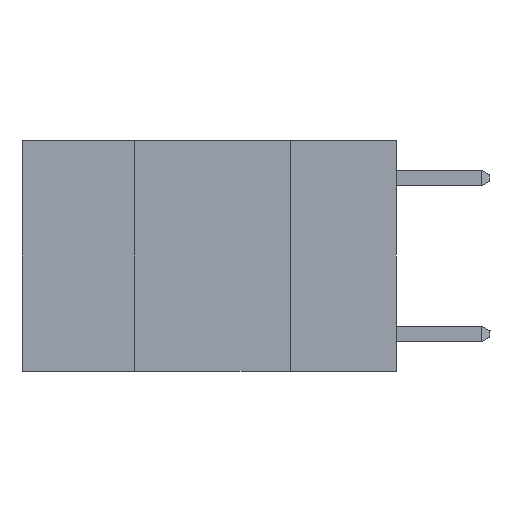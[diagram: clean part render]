
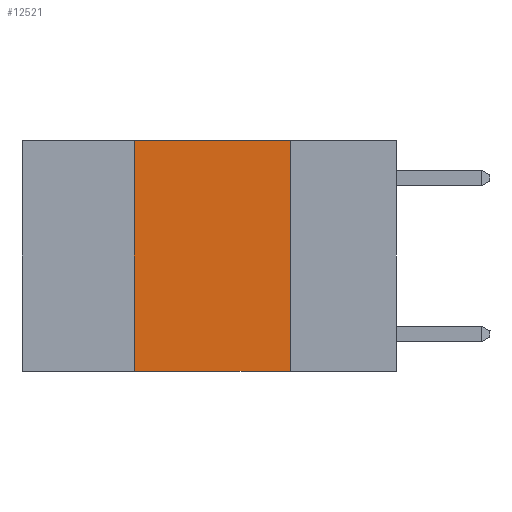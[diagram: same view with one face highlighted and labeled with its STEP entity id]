
A CAD part, left-side view. The second image highlights one B-rep face of the part: STEP entity #12521.
In plain terms, the highlighted planar face has unit normal (-1, 0, 0).
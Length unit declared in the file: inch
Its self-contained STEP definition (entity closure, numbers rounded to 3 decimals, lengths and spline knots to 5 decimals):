
#1039 = DIRECTION ( 'NONE',  ( 0., -1., 0. ) ) ;
#2225 = VECTOR ( 'NONE', #25345, 39.37008 ) ;
#4602 = DIRECTION ( 'NONE',  ( 0., -1., 0. ) ) ;
#4793 = EDGE_CURVE ( 'NONE', #11114, #27344, #6600, .T. ) ;
#6600 = LINE ( 'NONE', #28988, #23838 ) ;
#6808 = FACE_OUTER_BOUND ( 'NONE', #7672, .T. ) ;
#7672 = EDGE_LOOP ( 'NONE', ( #29712, #24950, #14705, #21653 ) ) ;
#9462 = PLANE ( 'NONE',  #22714 ) ;
#11114 = VERTEX_POINT ( 'NONE', #17862 ) ;
#11649 = CARTESIAN_POINT ( 'NONE',  ( 0., 0.17, -0.37 ) ) ;
#11840 = DIRECTION ( 'NONE',  ( 0., 0., -1. ) ) ;
#12386 = CARTESIAN_POINT ( 'NONE',  ( 0., 0.42, 0. ) ) ;
#12521 = ADVANCED_FACE ( 'NONE', ( #6808 ), #9462, .F. ) ;
#13565 = VECTOR ( 'NONE', #4602, 39.37008 ) ;
#13646 = VERTEX_POINT ( 'NONE', #23130 ) ;
#14705 = ORIENTED_EDGE ( 'NONE', *, *, #15365, .F. ) ;
#15365 = EDGE_CURVE ( 'NONE', #11114, #28292, #27159, .T. ) ;
#16125 = EDGE_CURVE ( 'NONE', #28292, #13646, #21261, .T. ) ;
#16358 = VECTOR ( 'NONE', #23430, 39.37008 ) ;
#17862 = CARTESIAN_POINT ( 'NONE',  ( 0., 0.42, -0.37 ) ) ;
#19428 = EDGE_CURVE ( 'NONE', #13646, #27344, #22568, .T. ) ;
#21086 = CARTESIAN_POINT ( 'NONE',  ( 0., 0.17, 0. ) ) ;
#21261 = LINE ( 'NONE', #30309, #13565 ) ;
#21653 = ORIENTED_EDGE ( 'NONE', *, *, #4793, .T. ) ;
#22568 = LINE ( 'NONE', #21086, #16358 ) ;
#22714 = AXIS2_PLACEMENT_3D ( 'NONE', #23493, #25834, #11840 ) ;
#23130 = CARTESIAN_POINT ( 'NONE',  ( 0., 0.17, 0. ) ) ;
#23430 = DIRECTION ( 'NONE',  ( 0., 0., -1. ) ) ;
#23493 = CARTESIAN_POINT ( 'NONE',  ( 0., 0.6, 0. ) ) ;
#23838 = VECTOR ( 'NONE', #1039, 39.37008 ) ;
#24950 = ORIENTED_EDGE ( 'NONE', *, *, #16125, .F. ) ;
#25345 = DIRECTION ( 'NONE',  ( 0., 0., 1. ) ) ;
#25834 = DIRECTION ( 'NONE',  ( 1., 0., 0. ) ) ;
#27159 = LINE ( 'NONE', #27709, #2225 ) ;
#27344 = VERTEX_POINT ( 'NONE', #11649 ) ;
#27709 = CARTESIAN_POINT ( 'NONE',  ( 0., 0.42, 0. ) ) ;
#28292 = VERTEX_POINT ( 'NONE', #12386 ) ;
#28988 = CARTESIAN_POINT ( 'NONE',  ( 0., 0.6, -0.37 ) ) ;
#29712 = ORIENTED_EDGE ( 'NONE', *, *, #19428, .F. ) ;
#30309 = CARTESIAN_POINT ( 'NONE',  ( 0., 0.6, 0. ) ) ;
